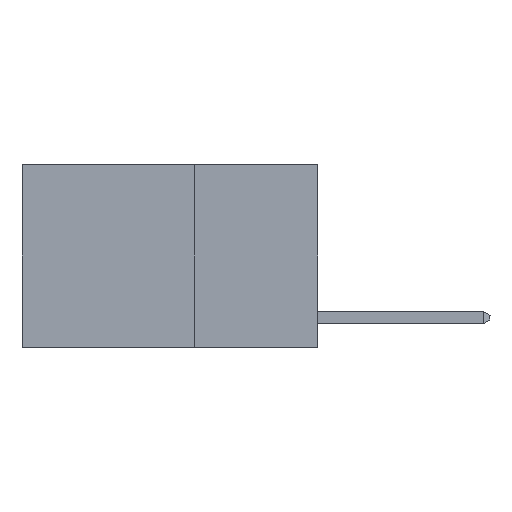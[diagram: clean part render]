
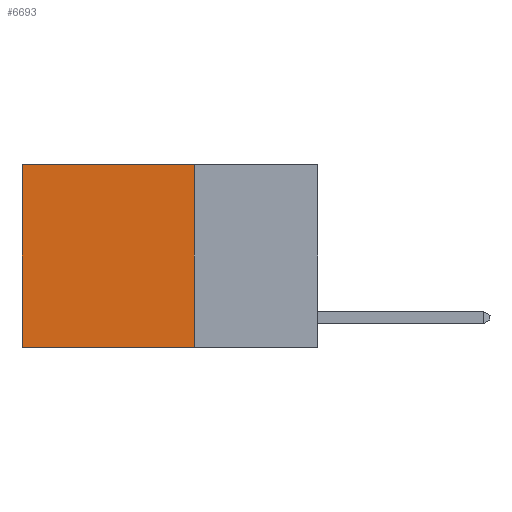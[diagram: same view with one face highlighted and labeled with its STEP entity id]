
A CAD part, left-side view. The second image highlights one B-rep face of the part: STEP entity #6693.
In plain terms, the highlighted planar face has unit normal (-1, 0, 0).
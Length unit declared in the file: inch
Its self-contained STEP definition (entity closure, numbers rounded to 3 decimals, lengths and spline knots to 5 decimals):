
#132 = DIRECTION ( 'NONE',  ( 1., 0., 0. ) ) ;
#551 = VECTOR ( 'NONE', #13718, 39.37008 ) ;
#1000 = ORIENTED_EDGE ( 'NONE', *, *, #15848, .T. ) ;
#3484 = LINE ( 'NONE', #6881, #551 ) ;
#3544 = DIRECTION ( 'NONE',  ( 0., 1., 0. ) ) ;
#4788 = VECTOR ( 'NONE', #14934, 39.37008 ) ;
#5203 = EDGE_LOOP ( 'NONE', ( #19403, #16670, #17976, #1000 ) ) ;
#5916 = CARTESIAN_POINT ( 'NONE',  ( 0.2625, 0.25, -0.37 ) ) ;
#6140 = CARTESIAN_POINT ( 'NONE',  ( 0.2625, 0.25, 0. ) ) ;
#6693 = ADVANCED_FACE ( 'NONE', ( #10163 ), #10492, .F. ) ;
#6710 = VERTEX_POINT ( 'NONE', #15624 ) ;
#6881 = CARTESIAN_POINT ( 'NONE',  ( 0.2625, 0.25, 0. ) ) ;
#7077 = VECTOR ( 'NONE', #3544, 39.37008 ) ;
#8381 = EDGE_CURVE ( 'NONE', #6710, #11679, #21559, .T. ) ;
#8718 = VECTOR ( 'NONE', #20057, 39.37008 ) ;
#8813 = CARTESIAN_POINT ( 'NONE',  ( 0.2625, 0.25, 0. ) ) ;
#9290 = VERTEX_POINT ( 'NONE', #5916 ) ;
#10163 = FACE_OUTER_BOUND ( 'NONE', #5203, .T. ) ;
#10201 = AXIS2_PLACEMENT_3D ( 'NONE', #8813, #132, #15648 ) ;
#10492 = PLANE ( 'NONE',  #10201 ) ;
#11679 = VERTEX_POINT ( 'NONE', #21753 ) ;
#12982 = LINE ( 'NONE', #13217, #8718 ) ;
#13217 = CARTESIAN_POINT ( 'NONE',  ( 0.2625, 0.25, 0. ) ) ;
#13718 = DIRECTION ( 'NONE',  ( 0., 0., -1. ) ) ;
#14934 = DIRECTION ( 'NONE',  ( 0., 0., -1. ) ) ;
#15288 = EDGE_CURVE ( 'NONE', #18383, #9290, #3484, .T. ) ;
#15624 = CARTESIAN_POINT ( 'NONE',  ( 0.2625, 0.6, 0. ) ) ;
#15648 = DIRECTION ( 'NONE',  ( 0., 0., -1. ) ) ;
#15848 = EDGE_CURVE ( 'NONE', #18383, #6710, #12982, .T. ) ;
#16670 = ORIENTED_EDGE ( 'NONE', *, *, #17373, .F. ) ;
#17373 = EDGE_CURVE ( 'NONE', #9290, #11679, #17477, .T. ) ;
#17477 = LINE ( 'NONE', #18957, #7077 ) ;
#17976 = ORIENTED_EDGE ( 'NONE', *, *, #15288, .F. ) ;
#18383 = VERTEX_POINT ( 'NONE', #6140 ) ;
#18957 = CARTESIAN_POINT ( 'NONE',  ( 0.2625, 0.25, -0.37 ) ) ;
#19403 = ORIENTED_EDGE ( 'NONE', *, *, #8381, .T. ) ;
#20057 = DIRECTION ( 'NONE',  ( 0., 1., 0. ) ) ;
#21453 = CARTESIAN_POINT ( 'NONE',  ( 0.2625, 0.6, 0. ) ) ;
#21559 = LINE ( 'NONE', #21453, #4788 ) ;
#21753 = CARTESIAN_POINT ( 'NONE',  ( 0.2625, 0.6, -0.37 ) ) ;
